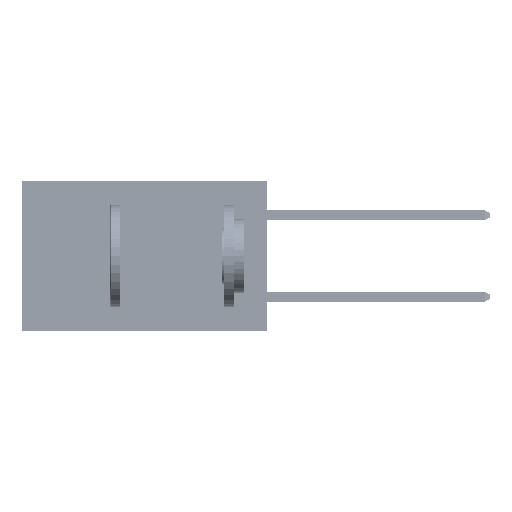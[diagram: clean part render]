
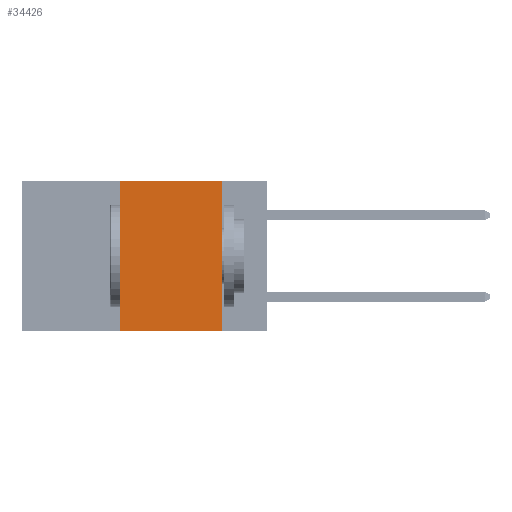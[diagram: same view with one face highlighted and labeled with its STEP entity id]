
A CAD part, left-side view. The second image highlights one B-rep face of the part: STEP entity #34426.
In plain terms, the highlighted planar face has unit normal (-1, 0, 0).
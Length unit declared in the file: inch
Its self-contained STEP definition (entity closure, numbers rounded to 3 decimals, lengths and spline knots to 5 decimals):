
#599 = CARTESIAN_POINT ( 'NONE',  ( 0., 0.11, 0. ) ) ;
#1106 = EDGE_CURVE ( 'NONE', #9202, #21229, #29339, .T. ) ;
#2166 = EDGE_CURVE ( 'NONE', #9202, #18625, #44599, .T. ) ;
#2487 = EDGE_CURVE ( 'NONE', #28204, #21229, #16909, .T. ) ;
#4825 = DIRECTION ( 'NONE',  ( 0., 0., -1. ) ) ;
#8887 = CARTESIAN_POINT ( 'NONE',  ( 0., 0.36, -0.37 ) ) ;
#9202 = VERTEX_POINT ( 'NONE', #8887 ) ;
#11086 = VECTOR ( 'NONE', #12795, 39.37008 ) ;
#12795 = DIRECTION ( 'NONE',  ( 0., -1., 0. ) ) ;
#14011 = EDGE_LOOP ( 'NONE', ( #43225, #36197, #41318, #52164 ) ) ;
#15340 = DIRECTION ( 'NONE',  ( 0., 0., 1. ) ) ;
#16909 = LINE ( 'NONE', #599, #48350 ) ;
#18006 = CARTESIAN_POINT ( 'NONE',  ( 0., 0.6, 0. ) ) ;
#18625 = VERTEX_POINT ( 'NONE', #24892 ) ;
#19973 = EDGE_CURVE ( 'NONE', #18625, #28204, #42599, .T. ) ;
#20209 = AXIS2_PLACEMENT_3D ( 'NONE', #18006, #46683, #22177 ) ;
#20325 = FACE_OUTER_BOUND ( 'NONE', #14011, .T. ) ;
#21229 = VERTEX_POINT ( 'NONE', #33073 ) ;
#22177 = DIRECTION ( 'NONE',  ( 0., 0., -1. ) ) ;
#23501 = CARTESIAN_POINT ( 'NONE',  ( 0., 0.36, 0. ) ) ;
#24892 = CARTESIAN_POINT ( 'NONE',  ( 0., 0.36, 0. ) ) ;
#28204 = VERTEX_POINT ( 'NONE', #42745 ) ;
#29339 = LINE ( 'NONE', #50064, #51079 ) ;
#33073 = CARTESIAN_POINT ( 'NONE',  ( 0., 0.11, -0.37 ) ) ;
#34426 = ADVANCED_FACE ( 'NONE', ( #20325 ), #42610, .F. ) ;
#36197 = ORIENTED_EDGE ( 'NONE', *, *, #19973, .F. ) ;
#37471 = CARTESIAN_POINT ( 'NONE',  ( 0., 0.6, 0. ) ) ;
#41318 = ORIENTED_EDGE ( 'NONE', *, *, #2166, .F. ) ;
#41874 = DIRECTION ( 'NONE',  ( 0., -1., 0. ) ) ;
#42599 = LINE ( 'NONE', #37471, #11086 ) ;
#42610 = PLANE ( 'NONE',  #20209 ) ;
#42745 = CARTESIAN_POINT ( 'NONE',  ( 0., 0.11, 0. ) ) ;
#43225 = ORIENTED_EDGE ( 'NONE', *, *, #2487, .F. ) ;
#43310 = VECTOR ( 'NONE', #15340, 39.37008 ) ;
#44599 = LINE ( 'NONE', #23501, #43310 ) ;
#46683 = DIRECTION ( 'NONE',  ( 1., 0., 0. ) ) ;
#48350 = VECTOR ( 'NONE', #4825, 39.37008 ) ;
#50064 = CARTESIAN_POINT ( 'NONE',  ( 0., 0.6, -0.37 ) ) ;
#51079 = VECTOR ( 'NONE', #41874, 39.37008 ) ;
#52164 = ORIENTED_EDGE ( 'NONE', *, *, #1106, .T. ) ;
